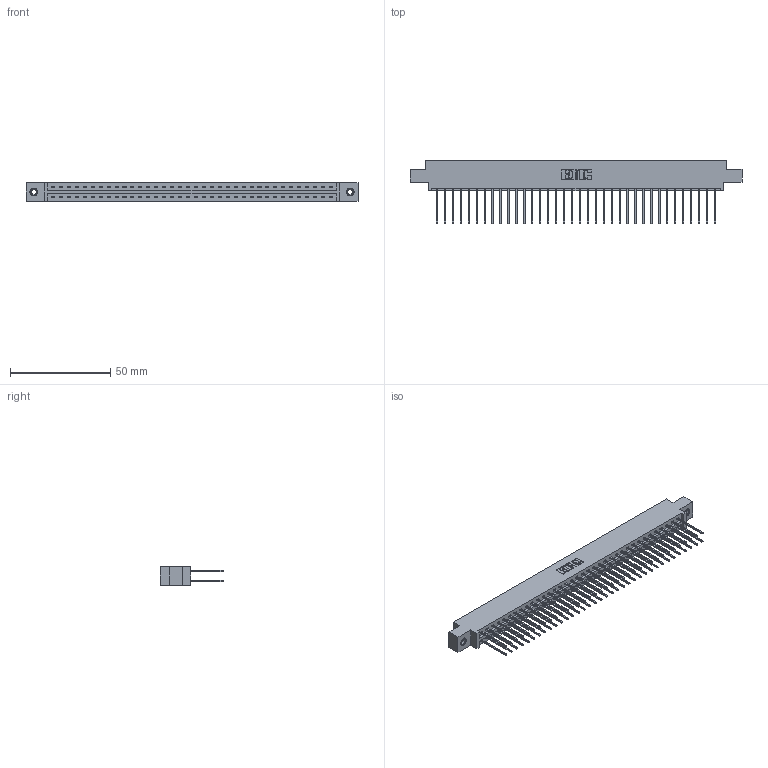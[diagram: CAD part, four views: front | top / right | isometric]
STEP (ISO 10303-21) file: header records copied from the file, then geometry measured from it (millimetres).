
FILE_DESCRIPTION (( 'STEP AP203' ), '1' );
FILE_NAME ('387-072-542-808.STEP', '2018-09-22T18:27:23', ( '' ), ( '' ), 'SwSTEP 2.0', 'SolidWorks 2016', '' );
FILE_SCHEMA (( 'CONFIG_CONTROL_DESIGN' ));
Length unit declared in the file: inch
Products named in the file (4): 345-292-001_345-293-142; 345-250-001_345-250-003-102; 387-072-542-808; 337 Part_0.170 Offset - 0.156 Dia-TI
Assembly tree (75 placements, depth 2):
  387-072-542-808
    337 Part_0.170 Offset - 0.156 Dia-TI
    345-292-001_345-293-142  x72
    345-250-001_345-250-003-102  x2
Bounding box: 165.66 x 31.63 x 9.4 mm (x, y, z)
Volume: 17590.2 mm3; surface area: 21632.5 mm2
Topology: 75 solids, 75 shells, 4066 faces, 12051 edges, 7930 vertices
Faces by surface type: plane 2842, cylinder 1208, cone 12, torus 4
Entity records: 30024 total; most frequent: CARTESIAN_POINT 5045, ORIENTED_EDGE 4974, DIRECTION 4333, EDGE_CURVE 2487, VECTOR 2339, LINE 2339, VERTEX_POINT 1652, AXIS2_PLACEMENT_3D 997
